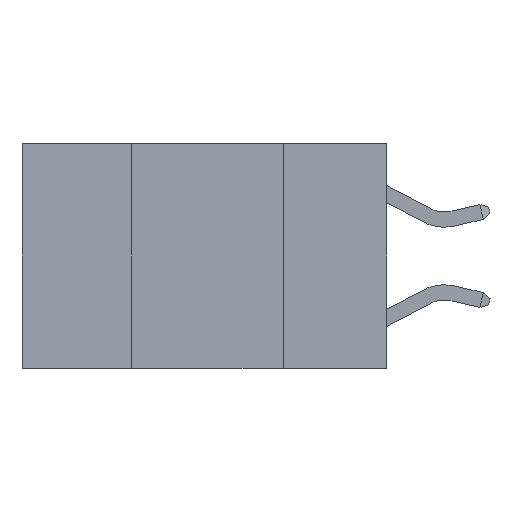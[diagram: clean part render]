
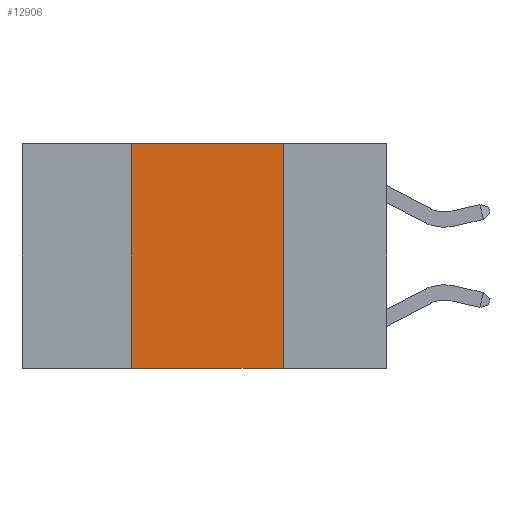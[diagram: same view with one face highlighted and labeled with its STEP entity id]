
A CAD part, left-side view. The second image highlights one B-rep face of the part: STEP entity #12906.
In plain terms, the highlighted planar face has unit normal (-1, 0, 0).
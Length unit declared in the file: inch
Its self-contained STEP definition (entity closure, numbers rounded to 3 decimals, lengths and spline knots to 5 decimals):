
#367 = ORIENTED_EDGE ( 'NONE', *, *, #11190, .F. ) ;
#586 = VECTOR ( 'NONE', #11301, 39.37008 ) ;
#751 = FACE_OUTER_BOUND ( 'NONE', #10107, .T. ) ;
#1261 = VECTOR ( 'NONE', #12764, 39.37008 ) ;
#1567 = CARTESIAN_POINT ( 'NONE',  ( 0., 0.17, 0. ) ) ;
#4300 = CARTESIAN_POINT ( 'NONE',  ( 0., 0.42, 0. ) ) ;
#4835 = CARTESIAN_POINT ( 'NONE',  ( 0., 0.6, 0. ) ) ;
#5352 = CARTESIAN_POINT ( 'NONE',  ( 0., 0.6, -0.37 ) ) ;
#6591 = LINE ( 'NONE', #5352, #14906 ) ;
#7059 = ORIENTED_EDGE ( 'NONE', *, *, #12128, .F. ) ;
#7178 = EDGE_CURVE ( 'NONE', #15425, #15505, #6591, .T. ) ;
#7194 = CARTESIAN_POINT ( 'NONE',  ( 0., 0.42, 0. ) ) ;
#7303 = CARTESIAN_POINT ( 'NONE',  ( 0., 0.42, -0.37 ) ) ;
#7456 = VERTEX_POINT ( 'NONE', #8981 ) ;
#8401 = LINE ( 'NONE', #9755, #586 ) ;
#8510 = LINE ( 'NONE', #1567, #1261 ) ;
#8525 = LINE ( 'NONE', #4300, #9787 ) ;
#8981 = CARTESIAN_POINT ( 'NONE',  ( 0., 0.17, 0. ) ) ;
#9653 = ORIENTED_EDGE ( 'NONE', *, *, #15790, .F. ) ;
#9755 = CARTESIAN_POINT ( 'NONE',  ( 0., 0.6, 0. ) ) ;
#9787 = VECTOR ( 'NONE', #9967, 39.37008 ) ;
#9967 = DIRECTION ( 'NONE',  ( 0., 0., 1. ) ) ;
#10107 = EDGE_LOOP ( 'NONE', ( #9653, #367, #7059, #15502 ) ) ;
#10830 = DIRECTION ( 'NONE',  ( 0., -1., 0. ) ) ;
#11190 = EDGE_CURVE ( 'NONE', #17182, #7456, #8401, .T. ) ;
#11301 = DIRECTION ( 'NONE',  ( 0., -1., 0. ) ) ;
#12128 = EDGE_CURVE ( 'NONE', #15425, #17182, #8525, .T. ) ;
#12764 = DIRECTION ( 'NONE',  ( 0., 0., -1. ) ) ;
#12906 = ADVANCED_FACE ( 'NONE', ( #751 ), #13128, .F. ) ;
#13128 = PLANE ( 'NONE',  #15891 ) ;
#13156 = CARTESIAN_POINT ( 'NONE',  ( 0., 0.17, -0.37 ) ) ;
#14906 = VECTOR ( 'NONE', #10830, 39.37008 ) ;
#15425 = VERTEX_POINT ( 'NONE', #7303 ) ;
#15502 = ORIENTED_EDGE ( 'NONE', *, *, #7178, .T. ) ;
#15505 = VERTEX_POINT ( 'NONE', #13156 ) ;
#15751 = DIRECTION ( 'NONE',  ( 0., 0., -1. ) ) ;
#15790 = EDGE_CURVE ( 'NONE', #7456, #15505, #8510, .T. ) ;
#15891 = AXIS2_PLACEMENT_3D ( 'NONE', #4835, #17109, #15751 ) ;
#17109 = DIRECTION ( 'NONE',  ( 1., 0., 0. ) ) ;
#17182 = VERTEX_POINT ( 'NONE', #7194 ) ;
